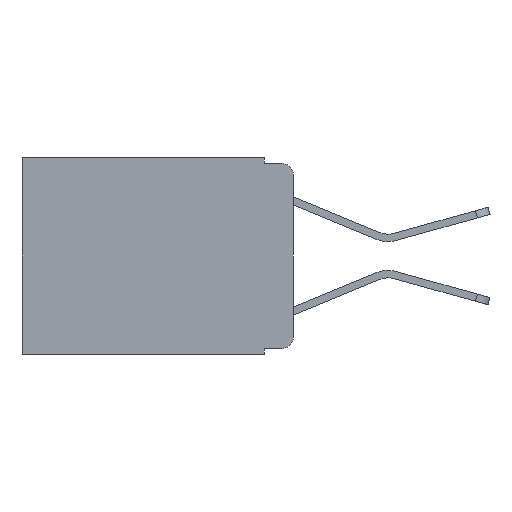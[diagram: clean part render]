
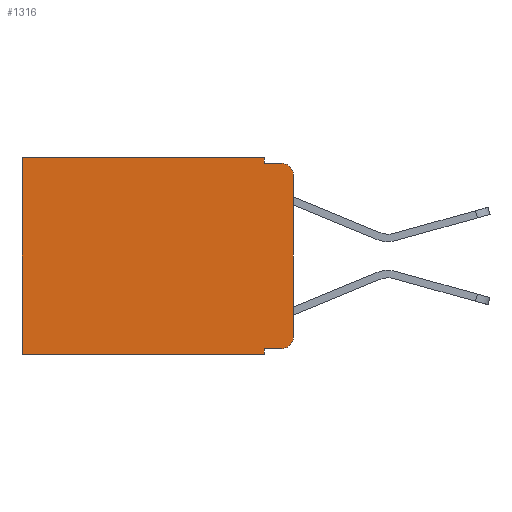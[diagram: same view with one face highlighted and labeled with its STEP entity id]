
A CAD part, left-side view. The second image highlights one B-rep face of the part: STEP entity #1316.
In plain terms, the highlighted planar face has unit normal (-1, 0, 0).
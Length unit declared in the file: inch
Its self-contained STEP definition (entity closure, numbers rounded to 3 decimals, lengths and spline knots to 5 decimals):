
#429 = DIRECTION ( 'NONE',  ( 0., 0., -1. ) ) ;
#954 = DIRECTION ( 'NONE',  ( 0., 0., -1. ) ) ;
#1241 = VERTEX_POINT ( 'NONE', #7058 ) ;
#1280 = LINE ( 'NONE', #12043, #17515 ) ;
#1298 = VECTOR ( 'NONE', #4629, 39.37008 ) ;
#1316 = ADVANCED_FACE ( 'NONE', ( #6903 ), #18538, .F. ) ;
#1574 = VERTEX_POINT ( 'NONE', #12803 ) ;
#2130 = DIRECTION ( 'NONE',  ( 0., 0., -1. ) ) ;
#2461 = VERTEX_POINT ( 'NONE', #19209 ) ;
#2950 = VECTOR ( 'NONE', #8993, 39.37008 ) ;
#3103 = VERTEX_POINT ( 'NONE', #15677 ) ;
#3189 = CARTESIAN_POINT ( 'NONE',  ( 0.298, 0.02, -0.313 ) ) ;
#3339 = VECTOR ( 'NONE', #6557, 39.37008 ) ;
#3680 = VECTOR ( 'NONE', #8287, 39.37008 ) ;
#3777 = DIRECTION ( 'NONE',  ( 0., 0., -1. ) ) ;
#3809 = CARTESIAN_POINT ( 'NONE',  ( 0.298, 0.02, -0.333 ) ) ;
#3847 = ORIENTED_EDGE ( 'NONE', *, *, #5905, .F. ) ;
#4005 = VERTEX_POINT ( 'NONE', #10180 ) ;
#4108 = VECTOR ( 'NONE', #17625, 39.37008 ) ;
#4629 = DIRECTION ( 'NONE',  ( 0., -1., 0. ) ) ;
#4836 = DIRECTION ( 'NONE',  ( 0., 0., -1. ) ) ;
#4916 = CARTESIAN_POINT ( 'NONE',  ( 0.298, 0.051, -0.01 ) ) ;
#5905 = EDGE_CURVE ( 'NONE', #19058, #1241, #8404, .T. ) ;
#6548 = ORIENTED_EDGE ( 'NONE', *, *, #17421, .T. ) ;
#6557 = DIRECTION ( 'NONE',  ( 0., -1., 0. ) ) ;
#6903 = FACE_OUTER_BOUND ( 'NONE', #16126, .T. ) ;
#7058 = CARTESIAN_POINT ( 'NONE',  ( 0.298, 0.051, -0.343 ) ) ;
#7063 = LINE ( 'NONE', #11304, #3339 ) ;
#7393 = LINE ( 'NONE', #17586, #3680 ) ;
#7938 = DIRECTION ( 'NONE',  ( 0., 0., -1. ) ) ;
#8287 = DIRECTION ( 'NONE',  ( 0., 0., -1. ) ) ;
#8404 = LINE ( 'NONE', #17816, #12053 ) ;
#8488 = AXIS2_PLACEMENT_3D ( 'NONE', #19275, #10019, #429 ) ;
#8685 = VERTEX_POINT ( 'NONE', #4916 ) ;
#8709 = EDGE_CURVE ( 'NONE', #8685, #18721, #7063, .T. ) ;
#8720 = ORIENTED_EDGE ( 'NONE', *, *, #8709, .F. ) ;
#8993 = DIRECTION ( 'NONE',  ( 0., 1., 0. ) ) ;
#10019 = DIRECTION ( 'NONE',  ( -1., 0., 0. ) ) ;
#10172 = VECTOR ( 'NONE', #7938, 39.37008 ) ;
#10180 = CARTESIAN_POINT ( 'NONE',  ( 0.298, 0., -0.313 ) ) ;
#10403 = ORIENTED_EDGE ( 'NONE', *, *, #13676, .T. ) ;
#10529 = ORIENTED_EDGE ( 'NONE', *, *, #16016, .T. ) ;
#10821 = EDGE_CURVE ( 'NONE', #14424, #8685, #7393, .T. ) ;
#11304 = CARTESIAN_POINT ( 'NONE',  ( 0.298, 0.051, -0.01 ) ) ;
#11980 = AXIS2_PLACEMENT_3D ( 'NONE', #15558, #16004, #3777 ) ;
#12043 = CARTESIAN_POINT ( 'NONE',  ( 0.298, 0.473, 0. ) ) ;
#12053 = VECTOR ( 'NONE', #2130, 39.37008 ) ;
#12064 = CARTESIAN_POINT ( 'NONE',  ( 0.298, 0.02, -0.01 ) ) ;
#12421 = ORIENTED_EDGE ( 'NONE', *, *, #12615, .T. ) ;
#12615 = EDGE_CURVE ( 'NONE', #15220, #4005, #14954, .T. ) ;
#12690 = CARTESIAN_POINT ( 'NONE',  ( 0.298, 0.051, 0. ) ) ;
#12803 = CARTESIAN_POINT ( 'NONE',  ( 0.298, 0.473, 0. ) ) ;
#13389 = ORIENTED_EDGE ( 'NONE', *, *, #20123, .F. ) ;
#13676 = EDGE_CURVE ( 'NONE', #19058, #15220, #13938, .T. ) ;
#13821 = ORIENTED_EDGE ( 'NONE', *, *, #19529, .F. ) ;
#13938 = LINE ( 'NONE', #15582, #1298 ) ;
#14129 = ORIENTED_EDGE ( 'NONE', *, *, #16662, .T. ) ;
#14175 = CARTESIAN_POINT ( 'NONE',  ( 0.298, 0., 0. ) ) ;
#14234 = DIRECTION ( 'NONE',  ( -1., 0., 0. ) ) ;
#14424 = VERTEX_POINT ( 'NONE', #12690 ) ;
#14954 = CIRCLE ( 'NONE', #15664, 0.02 ) ;
#15049 = CIRCLE ( 'NONE', #8488, 0.02 ) ;
#15220 = VERTEX_POINT ( 'NONE', #3809 ) ;
#15558 = CARTESIAN_POINT ( 'NONE',  ( 0.298, 0., 0. ) ) ;
#15582 = CARTESIAN_POINT ( 'NONE',  ( 0.298, 0.051, -0.333 ) ) ;
#15664 = AXIS2_PLACEMENT_3D ( 'NONE', #3189, #14234, #4836 ) ;
#15677 = CARTESIAN_POINT ( 'NONE',  ( 0.298, 0., -0.03 ) ) ;
#16004 = DIRECTION ( 'NONE',  ( 1., 0., 0. ) ) ;
#16016 = EDGE_CURVE ( 'NONE', #3103, #18721, #15049, .T. ) ;
#16094 = CARTESIAN_POINT ( 'NONE',  ( 0.298, 0., 0. ) ) ;
#16126 = EDGE_LOOP ( 'NONE', ( #13821, #10529, #8720, #17862, #14129, #6548, #13389, #3847, #10403, #12421 ) ) ;
#16585 = LINE ( 'NONE', #16094, #4108 ) ;
#16662 = EDGE_CURVE ( 'NONE', #14424, #1574, #16585, .T. ) ;
#16714 = CARTESIAN_POINT ( 'NONE',  ( 0.298, 0., -0.343 ) ) ;
#17421 = EDGE_CURVE ( 'NONE', #1574, #2461, #1280, .T. ) ;
#17515 = VECTOR ( 'NONE', #954, 39.37008 ) ;
#17586 = CARTESIAN_POINT ( 'NONE',  ( 0.298, 0.051, 0. ) ) ;
#17625 = DIRECTION ( 'NONE',  ( 0., 1., 0. ) ) ;
#17816 = CARTESIAN_POINT ( 'NONE',  ( 0.298, 0.051, 0. ) ) ;
#17862 = ORIENTED_EDGE ( 'NONE', *, *, #10821, .F. ) ;
#18509 = CARTESIAN_POINT ( 'NONE',  ( 0.298, 0.051, -0.333 ) ) ;
#18538 = PLANE ( 'NONE',  #11980 ) ;
#18639 = LINE ( 'NONE', #16714, #2950 ) ;
#18721 = VERTEX_POINT ( 'NONE', #12064 ) ;
#18873 = LINE ( 'NONE', #14175, #10172 ) ;
#19058 = VERTEX_POINT ( 'NONE', #18509 ) ;
#19209 = CARTESIAN_POINT ( 'NONE',  ( 0.298, 0.473, -0.343 ) ) ;
#19275 = CARTESIAN_POINT ( 'NONE',  ( 0.298, 0.02, -0.03 ) ) ;
#19529 = EDGE_CURVE ( 'NONE', #3103, #4005, #18873, .T. ) ;
#20123 = EDGE_CURVE ( 'NONE', #1241, #2461, #18639, .T. ) ;
